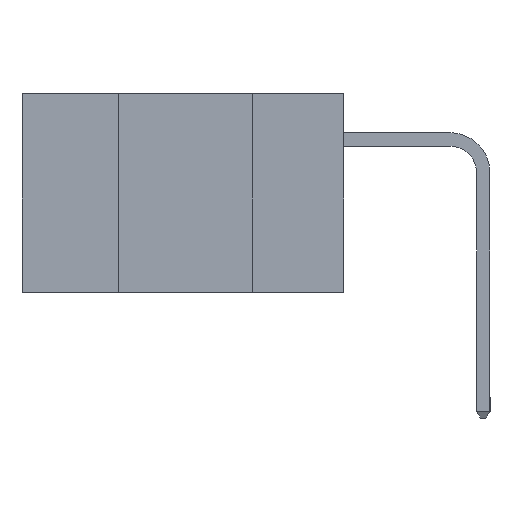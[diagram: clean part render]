
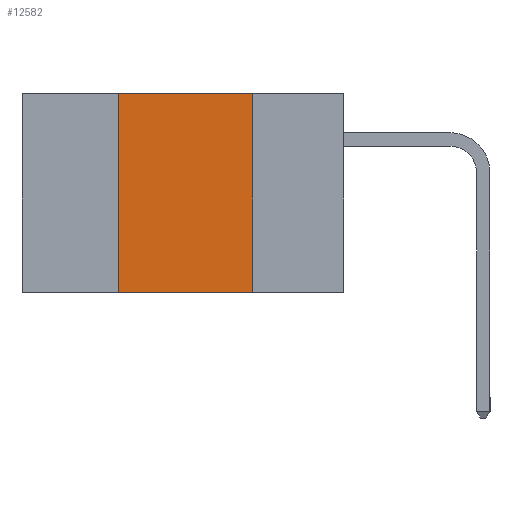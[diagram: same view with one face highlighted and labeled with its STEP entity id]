
A CAD part, left-side view. The second image highlights one B-rep face of the part: STEP entity #12582.
In plain terms, the highlighted planar face has unit normal (-1, 0, 0).
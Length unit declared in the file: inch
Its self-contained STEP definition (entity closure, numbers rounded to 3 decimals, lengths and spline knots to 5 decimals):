
#295 = LINE ( 'NONE', #6404, #18021 ) ;
#357 = VERTEX_POINT ( 'NONE', #11103 ) ;
#370 = CARTESIAN_POINT ( 'NONE',  ( 0., 0.17, -0.37 ) ) ;
#554 = VERTEX_POINT ( 'NONE', #22025 ) ;
#1679 = VECTOR ( 'NONE', #19120, 39.37008 ) ;
#2119 = ORIENTED_EDGE ( 'NONE', *, *, #12441, .F. ) ;
#2285 = VERTEX_POINT ( 'NONE', #370 ) ;
#3172 = DIRECTION ( 'NONE',  ( 1., 0., 0. ) ) ;
#3868 = AXIS2_PLACEMENT_3D ( 'NONE', #13837, #3172, #15577 ) ;
#5652 = CARTESIAN_POINT ( 'NONE',  ( 0., 0.17, -0.37 ) ) ;
#6170 = EDGE_LOOP ( 'NONE', ( #20157, #20477, #2119, #19862 ) ) ;
#6404 = CARTESIAN_POINT ( 'NONE',  ( 0., 0.42, -0.37 ) ) ;
#9427 = LINE ( 'NONE', #15792, #14106 ) ;
#9990 = DIRECTION ( 'NONE',  ( 0., 0., 1. ) ) ;
#10219 = EDGE_CURVE ( 'NONE', #357, #12371, #9427, .T. ) ;
#11103 = CARTESIAN_POINT ( 'NONE',  ( 0., 0.42, 0. ) ) ;
#12141 = EDGE_CURVE ( 'NONE', #12371, #2285, #19840, .T. ) ;
#12371 = VERTEX_POINT ( 'NONE', #15047 ) ;
#12441 = EDGE_CURVE ( 'NONE', #554, #357, #295, .T. ) ;
#12582 = ADVANCED_FACE ( 'NONE', ( #20321 ), #22176, .F. ) ;
#13837 = CARTESIAN_POINT ( 'NONE',  ( 0., 0.6, 0. ) ) ;
#14106 = VECTOR ( 'NONE', #15808, 39.37008 ) ;
#15047 = CARTESIAN_POINT ( 'NONE',  ( 0., 0.17, 0. ) ) ;
#15577 = DIRECTION ( 'NONE',  ( 0., 0., -1. ) ) ;
#15725 = CARTESIAN_POINT ( 'NONE',  ( 0., 0.6, -0.37 ) ) ;
#15792 = CARTESIAN_POINT ( 'NONE',  ( 0., 0.6, 0. ) ) ;
#15808 = DIRECTION ( 'NONE',  ( 0., -1., 0. ) ) ;
#16200 = DIRECTION ( 'NONE',  ( 0., 0., -1. ) ) ;
#16386 = LINE ( 'NONE', #15725, #1679 ) ;
#18021 = VECTOR ( 'NONE', #9990, 39.37008 ) ;
#19120 = DIRECTION ( 'NONE',  ( 0., -1., 0. ) ) ;
#19334 = VECTOR ( 'NONE', #16200, 39.37008 ) ;
#19840 = LINE ( 'NONE', #5652, #19334 ) ;
#19862 = ORIENTED_EDGE ( 'NONE', *, *, #21114, .T. ) ;
#20157 = ORIENTED_EDGE ( 'NONE', *, *, #12141, .F. ) ;
#20321 = FACE_OUTER_BOUND ( 'NONE', #6170, .T. ) ;
#20477 = ORIENTED_EDGE ( 'NONE', *, *, #10219, .F. ) ;
#21114 = EDGE_CURVE ( 'NONE', #554, #2285, #16386, .T. ) ;
#22025 = CARTESIAN_POINT ( 'NONE',  ( 0., 0.42, -0.37 ) ) ;
#22176 = PLANE ( 'NONE',  #3868 ) ;
